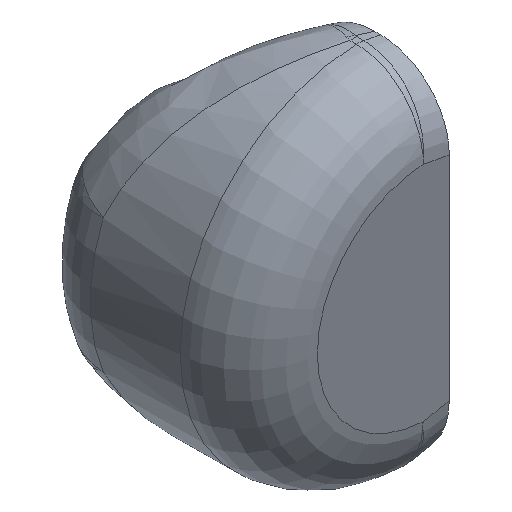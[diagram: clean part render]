
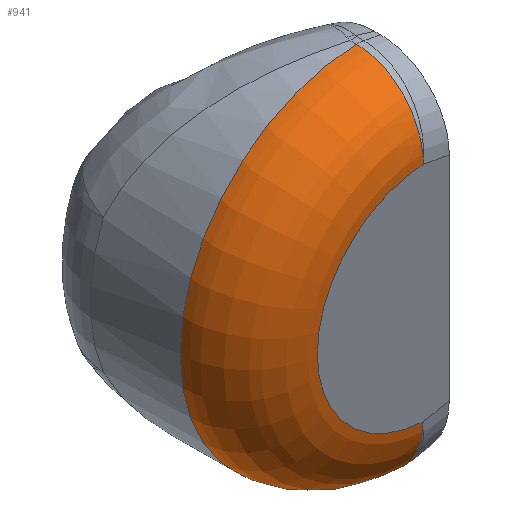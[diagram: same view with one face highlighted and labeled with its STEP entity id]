
A CAD part, isometric view. The second image highlights one B-rep face of the part: STEP entity #941.
In plain terms, the highlighted toroidal (fillet/blend) face has major radius 16.269 mm and minor radius 10 mm.
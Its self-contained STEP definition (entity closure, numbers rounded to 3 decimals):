
#31 = CARTESIAN_POINT ( 'NONE',  ( -295.176, -58.188, 29.918 ) ) ;
#36 = CARTESIAN_POINT ( 'NONE',  ( -295.391, -63.794, 23.064 ) ) ;
#73 = CARTESIAN_POINT ( 'NONE',  ( -295.195, -59.06, -20.373 ) ) ;
#76 = CARTESIAN_POINT ( 'NONE',  ( -295.407, -63.969, -13.008 ) ) ;
#146 = CARTESIAN_POINT ( 'NONE',  ( -295.195, -59.06, 29.468 ) ) ;
#151 = CARTESIAN_POINT ( 'NONE',  ( -295.407, -63.969, 22.102 ) ) ;
#178 = CARTESIAN_POINT ( 'NONE',  ( -295.137, -54.049, -21.715 ) ) ;
#186 = CARTESIAN_POINT ( 'NONE',  ( -295.224, -60.162, -19.653 ) ) ;
#190 = CARTESIAN_POINT ( 'NONE',  ( -295.419, -64.049, -12.028 ) ) ;
#199 = CARTESIAN_POINT ( 'NONE',  ( -294.564, -54.049, 4.547 ) ) ;
#204 = DIRECTION ( 'NONE',  ( -1., 0., 0. ) ) ;
#230 = B_SPLINE_CURVE_WITH_KNOTS ( 'NONE', 3,
 ( #178, #767, #511, #1400, #635, #1487, #772, #73, #909, #186, #1041, #290, #1163, #397, #1294, #514, #1402, #639, #1490, #778, #76, #914, #190, #1044 ),
 .UNSPECIFIED., .F., .F.,
 ( 4, 2, 2, 2, 2, 2, 2, 2, 2, 2, 2, 4 ),
 ( 0., 0.002, 0.004, 0.005, 0.006, 0.008, 0.01, 0.012, 0.013, 0.014, 0.015, 0.016 ),
 .UNSPECIFIED. ) ;
#253 = CARTESIAN_POINT ( 'NONE',  ( -295.224, -60.162, 28.748 ) ) ;
#259 = CARTESIAN_POINT ( 'NONE',  ( -295.419, -64.049, 21.123 ) ) ;
#281 = CARTESIAN_POINT ( 'NONE',  ( -294.564, -54.049, 4.547 ) ) ;
#285 = AXIS2_PLACEMENT_3D ( 'NONE', #281, #1152, #389 ) ;
#290 = CARTESIAN_POINT ( 'NONE',  ( -295.273, -61.587, -18.314 ) ) ;
#306 = AXIS2_PLACEMENT_3D ( 'NONE', #1276, #504, #1392 ) ;
#340 = CARTESIAN_POINT ( 'NONE',  ( -295.422, -64.049, 20.794 ) ) ;
#345 = CARTESIAN_POINT ( 'NONE',  ( -295.422, -64.049, -11.699 ) ) ;
#351 = CARTESIAN_POINT ( 'NONE',  ( -295.273, -61.587, 27.409 ) ) ;
#389 = DIRECTION ( 'NONE',  ( -1., 0., 0. ) ) ;
#397 = CARTESIAN_POINT ( 'NONE',  ( -295.325, -62.732, -16.711 ) ) ;
#462 = CIRCLE ( 'NONE', #285, 26.269 ) ;
#467 = CARTESIAN_POINT ( 'NONE',  ( -295.137, -54.049, 30.81 ) ) ;
#473 = CARTESIAN_POINT ( 'NONE',  ( -295.325, -62.732, 25.806 ) ) ;
#478 = CIRCLE ( 'NONE', #306, 16.269 ) ;
#504 = DIRECTION ( 'NONE',  ( 0., -1., 0. ) ) ;
#511 = CARTESIAN_POINT ( 'NONE',  ( -295.14, -55.364, -21.65 ) ) ;
#514 = CARTESIAN_POINT ( 'NONE',  ( -295.364, -63.414, -15.226 ) ) ;
#535 = DIRECTION ( 'NONE',  ( 0., 1., 0. ) ) ;
#547 = TOROIDAL_SURFACE ( 'NONE', #698, 16.269, 10. ) ;
#584 = CARTESIAN_POINT ( 'NONE',  ( -295.14, -55.364, 30.745 ) ) ;
#591 = CARTESIAN_POINT ( 'NONE',  ( -295.364, -63.414, 24.321 ) ) ;
#635 = CARTESIAN_POINT ( 'NONE',  ( -295.16, -57.286, -21.199 ) ) ;
#639 = CARTESIAN_POINT ( 'NONE',  ( -295.384, -63.715, -14.286 ) ) ;
#645 = B_SPLINE_CURVE_WITH_KNOTS ( 'NONE', 3,
 ( #467, #1364, #584, #1455, #720, #31, #850, #146, #994, #253, #1111, #351, #1241, #473, #1370, #591, #1459, #727, #36, #859, #151, #1001, #259, #1116 ),
 .UNSPECIFIED., .F., .F.,
 ( 4, 2, 2, 2, 2, 2, 2, 2, 2, 2, 2, 4 ),
 ( 0., 0.002, 0.004, 0.005, 0.006, 0.008, 0.01, 0.012, 0.013, 0.014, 0.015, 0.016 ),
 .UNSPECIFIED. ) ;
#698 = AXIS2_PLACEMENT_3D ( 'NONE', #199, #535, #204 ) ;
#720 = CARTESIAN_POINT ( 'NONE',  ( -295.16, -57.286, 30.294 ) ) ;
#727 = CARTESIAN_POINT ( 'NONE',  ( -295.384, -63.715, 23.381 ) ) ;
#767 = CARTESIAN_POINT ( 'NONE',  ( -295.137, -54.71, -21.715 ) ) ;
#772 = CARTESIAN_POINT ( 'NONE',  ( -295.182, -58.483, -20.683 ) ) ;
#778 = CARTESIAN_POINT ( 'NONE',  ( -295.402, -63.921, -13.33 ) ) ;
#835 = FACE_OUTER_BOUND ( 'NONE', #1071, .T. ) ;
#844 = CARTESIAN_POINT ( 'NONE',  ( -295.137, -54.049, 30.81 ) ) ;
#850 = CARTESIAN_POINT ( 'NONE',  ( -295.182, -58.483, 29.778 ) ) ;
#859 = CARTESIAN_POINT ( 'NONE',  ( -295.402, -63.921, 22.425 ) ) ;
#909 = CARTESIAN_POINT ( 'NONE',  ( -295.202, -59.345, -20.202 ) ) ;
#914 = CARTESIAN_POINT ( 'NONE',  ( -295.415, -64.033, -12.357 ) ) ;
#941 = ADVANCED_FACE ( 'NONE', ( #835 ), #547, .T. ) ;
#994 = CARTESIAN_POINT ( 'NONE',  ( -295.202, -59.345, 29.297 ) ) ;
#1001 = CARTESIAN_POINT ( 'NONE',  ( -295.415, -64.033, 21.452 ) ) ;
#1041 = CARTESIAN_POINT ( 'NONE',  ( -295.24, -60.665, -19.239 ) ) ;
#1044 = CARTESIAN_POINT ( 'NONE',  ( -295.422, -64.049, -11.699 ) ) ;
#1071 = EDGE_LOOP ( 'NONE', ( #1325, #1328, #1340, #1349 ) ) ;
#1111 = CARTESIAN_POINT ( 'NONE',  ( -295.24, -60.665, 28.334 ) ) ;
#1116 = CARTESIAN_POINT ( 'NONE',  ( -295.422, -64.049, 20.794 ) ) ;
#1117 = VERTEX_POINT ( 'NONE', #340 ) ;
#1152 = DIRECTION ( 'NONE',  ( 0., 1., 0. ) ) ;
#1163 = CARTESIAN_POINT ( 'NONE',  ( -295.291, -62.008, -17.798 ) ) ;
#1223 = VERTEX_POINT ( 'NONE', #345 ) ;
#1226 = VERTEX_POINT ( 'NONE', #844 ) ;
#1233 = EDGE_CURVE ( 'NONE', #1226, #1117, #645, .T. ) ;
#1235 = CARTESIAN_POINT ( 'NONE',  ( -295.137, -54.049, -21.715 ) ) ;
#1241 = CARTESIAN_POINT ( 'NONE',  ( -295.291, -62.008, 26.893 ) ) ;
#1243 = VERTEX_POINT ( 'NONE', #1235 ) ;
#1276 = CARTESIAN_POINT ( 'NONE',  ( -294.564, -64.049, 4.547 ) ) ;
#1294 = CARTESIAN_POINT ( 'NONE',  ( -295.341, -63.038, -16.136 ) ) ;
#1325 = ORIENTED_EDGE ( 'NONE', *, *, #1432, .T. ) ;
#1328 = ORIENTED_EDGE ( 'NONE', *, *, #1382, .F. ) ;
#1340 = ORIENTED_EDGE ( 'NONE', *, *, #1233, .F. ) ;
#1349 = ORIENTED_EDGE ( 'NONE', *, *, #1393, .F. ) ;
#1364 = CARTESIAN_POINT ( 'NONE',  ( -295.137, -54.71, 30.81 ) ) ;
#1370 = CARTESIAN_POINT ( 'NONE',  ( -295.341, -63.038, 25.231 ) ) ;
#1382 = EDGE_CURVE ( 'NONE', #1117, #1223, #478, .T. ) ;
#1392 = DIRECTION ( 'NONE',  ( -1., 0., 0. ) ) ;
#1393 = EDGE_CURVE ( 'NONE', #1243, #1226, #462, .T. ) ;
#1400 = CARTESIAN_POINT ( 'NONE',  ( -295.151, -56.659, -21.391 ) ) ;
#1402 = CARTESIAN_POINT ( 'NONE',  ( -295.371, -63.526, -14.914 ) ) ;
#1432 = EDGE_CURVE ( 'NONE', #1243, #1223, #230, .T. ) ;
#1455 = CARTESIAN_POINT ( 'NONE',  ( -295.151, -56.659, 30.486 ) ) ;
#1459 = CARTESIAN_POINT ( 'NONE',  ( -295.371, -63.526, 24.009 ) ) ;
#1487 = CARTESIAN_POINT ( 'NONE',  ( -295.176, -58.188, -20.823 ) ) ;
#1490 = CARTESIAN_POINT ( 'NONE',  ( -295.391, -63.794, -13.969 ) ) ;
